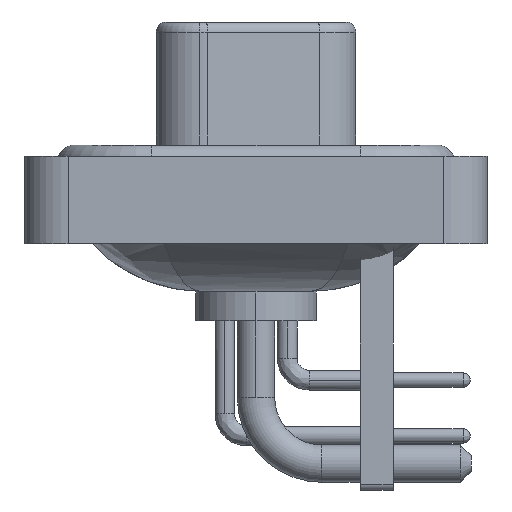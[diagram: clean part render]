
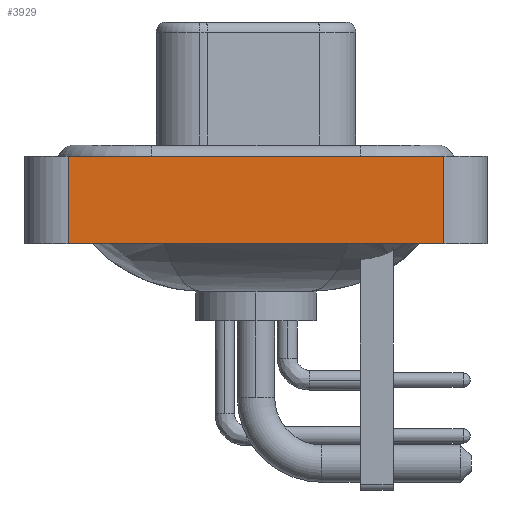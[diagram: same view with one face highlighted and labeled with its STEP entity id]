
A CAD part, left-side view. The second image highlights one B-rep face of the part: STEP entity #3929.
In plain terms, the highlighted planar face has unit normal (-1, 0, 0).
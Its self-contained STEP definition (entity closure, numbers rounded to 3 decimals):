
#896 = DIRECTION ( 'NONE',  ( 0., -1., 0. ) ) ;
#955 = EDGE_CURVE ( 'NONE', #15133, #25043, #17577, .T. ) ;
#2171 = VERTEX_POINT ( 'NONE', #4619 ) ;
#3559 = DIRECTION ( 'NONE',  ( 0., 0., 1. ) ) ;
#3929 = ADVANCED_FACE ( 'NONE', ( #26600 ), #7148, .T. ) ;
#3965 = AXIS2_PLACEMENT_3D ( 'NONE', #24473, #13647, #22331 ) ;
#4619 = CARTESIAN_POINT ( 'NONE',  ( -7.35, 8.55, 0.4 ) ) ;
#4873 = VECTOR ( 'NONE', #19321, 1000. ) ;
#5252 = CARTESIAN_POINT ( 'NONE',  ( -7.35, 8.55, -3.6 ) ) ;
#5532 = CARTESIAN_POINT ( 'NONE',  ( -7.35, 8.55, -3.6 ) ) ;
#5891 = LINE ( 'NONE', #19177, #4873 ) ;
#7148 = PLANE ( 'NONE',  #3965 ) ;
#7444 = CARTESIAN_POINT ( 'NONE',  ( -7.35, -8.55, -3.6 ) ) ;
#8438 = EDGE_CURVE ( 'NONE', #25043, #16013, #17774, .T. ) ;
#8887 = ORIENTED_EDGE ( 'NONE', *, *, #955, .T. ) ;
#9173 = VECTOR ( 'NONE', #896, 1000. ) ;
#11262 = EDGE_CURVE ( 'NONE', #2171, #16013, #5891, .T. ) ;
#11360 = EDGE_LOOP ( 'NONE', ( #26306, #21398, #20459, #8887 ) ) ;
#12005 = VECTOR ( 'NONE', #3559, 1000. ) ;
#13647 = DIRECTION ( 'NONE',  ( -1., 0., 0. ) ) ;
#15133 = VERTEX_POINT ( 'NONE', #5252 ) ;
#15145 = EDGE_CURVE ( 'NONE', #15133, #2171, #20414, .T. ) ;
#15457 = CARTESIAN_POINT ( 'NONE',  ( -7.35, -8.55, -3.6 ) ) ;
#15789 = DIRECTION ( 'NONE',  ( 0., 0., 1. ) ) ;
#16013 = VERTEX_POINT ( 'NONE', #25302 ) ;
#17577 = LINE ( 'NONE', #15457, #9173 ) ;
#17774 = LINE ( 'NONE', #7444, #26420 ) ;
#19177 = CARTESIAN_POINT ( 'NONE',  ( -7.35, -8.55, 0.4 ) ) ;
#19321 = DIRECTION ( 'NONE',  ( 0., -1., 0. ) ) ;
#20414 = LINE ( 'NONE', #5532, #12005 ) ;
#20459 = ORIENTED_EDGE ( 'NONE', *, *, #15145, .F. ) ;
#21398 = ORIENTED_EDGE ( 'NONE', *, *, #11262, .F. ) ;
#21966 = CARTESIAN_POINT ( 'NONE',  ( -7.35, -8.55, -3.6 ) ) ;
#22331 = DIRECTION ( 'NONE',  ( 0., 0., 1. ) ) ;
#24473 = CARTESIAN_POINT ( 'NONE',  ( -7.35, -8.55, -3.6 ) ) ;
#25043 = VERTEX_POINT ( 'NONE', #21966 ) ;
#25302 = CARTESIAN_POINT ( 'NONE',  ( -7.35, -8.55, 0.4 ) ) ;
#26306 = ORIENTED_EDGE ( 'NONE', *, *, #8438, .T. ) ;
#26420 = VECTOR ( 'NONE', #15789, 1000. ) ;
#26600 = FACE_OUTER_BOUND ( 'NONE', #11360, .T. ) ;
